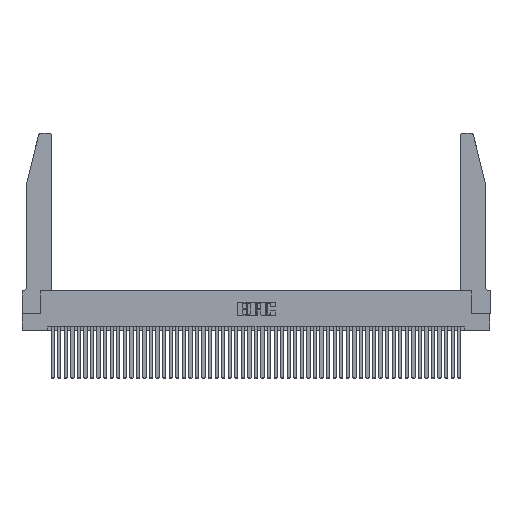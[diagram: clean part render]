
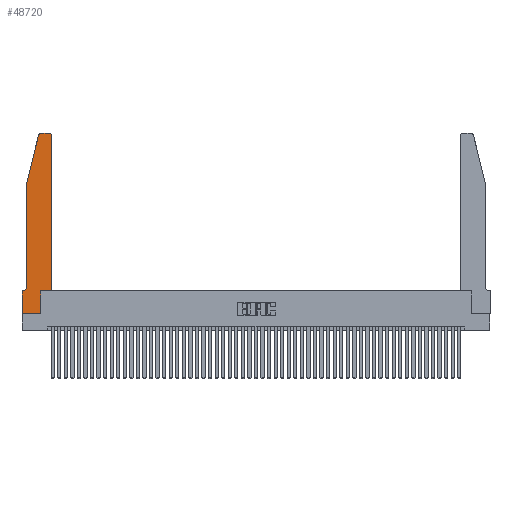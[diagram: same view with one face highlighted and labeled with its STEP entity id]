
A CAD part, top view. The second image highlights one B-rep face of the part: STEP entity #48720.
In plain terms, the highlighted planar face has unit normal (0, 0, 1).
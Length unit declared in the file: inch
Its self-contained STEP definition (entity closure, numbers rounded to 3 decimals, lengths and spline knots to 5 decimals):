
#128 = DIRECTION ( 'NONE',  ( 1., 0., 0. ) ) ;
#331 = CARTESIAN_POINT ( 'NONE',  ( 0.4505, 0.35, 0.37 ) ) ;
#742 = DIRECTION ( 'NONE',  ( -1., 0., 0. ) ) ;
#1206 = DIRECTION ( 'NONE',  ( 0., 1., 0. ) ) ;
#2209 = EDGE_CURVE ( 'NONE', #40006, #32432, #47138, .T. ) ;
#3001 = CARTESIAN_POINT ( 'NONE',  ( 0.0755, 2., 0.37 ) ) ;
#3090 = DIRECTION ( 'NONE',  ( 0., 0., 1. ) ) ;
#4704 = ORIENTED_EDGE ( 'NONE', *, *, #40652, .T. ) ;
#4999 = LINE ( 'NONE', #37681, #24915 ) ;
#5500 = DIRECTION ( 'NONE',  ( 1., 0., 0. ) ) ;
#5932 = AXIS2_PLACEMENT_3D ( 'NONE', #47526, #24015, #128 ) ;
#6295 = CARTESIAN_POINT ( 'NONE',  ( 0.284, 2.75, 0.37 ) ) ;
#7671 = CARTESIAN_POINT ( 'NONE',  ( 0.4505, 2.72, 0.37 ) ) ;
#7992 = VECTOR ( 'NONE', #13458, 39.37008 ) ;
#8046 = CARTESIAN_POINT ( 'NONE',  ( 0.0055, 0.42, 0.37 ) ) ;
#9437 = CARTESIAN_POINT ( 'NONE',  ( 0.0055, 0.35, 0.37 ) ) ;
#9988 = DIRECTION ( 'NONE',  ( 1., 0., 0. ) ) ;
#10695 = EDGE_CURVE ( 'NONE', #36535, #32628, #16369, .T. ) ;
#12051 = DIRECTION ( 'NONE',  ( -1., 0., 0. ) ) ;
#13458 = DIRECTION ( 'NONE',  ( -0.239, -0.971, 0. ) ) ;
#13918 = VERTEX_POINT ( 'NONE', #31488 ) ;
#13944 = EDGE_CURVE ( 'NONE', #13918, #24894, #30889, .T. ) ;
#14891 = CIRCLE ( 'NONE', #5932, 0.03 ) ;
#16247 = DIRECTION ( 'NONE',  ( 0., 1., 0. ) ) ;
#16369 = LINE ( 'NONE', #331, #21936 ) ;
#16769 = VECTOR ( 'NONE', #1206, 39.37008 ) ;
#17082 = CARTESIAN_POINT ( 'NONE',  ( 0.2865, 0., 0.37 ) ) ;
#17313 = ORIENTED_EDGE ( 'NONE', *, *, #24351, .T. ) ;
#17375 = DIRECTION ( 'NONE',  ( 0., 0., 1. ) ) ;
#17654 = ORIENTED_EDGE ( 'NONE', *, *, #47151, .T. ) ;
#17729 = ORIENTED_EDGE ( 'NONE', *, *, #24522, .T. ) ;
#20104 = AXIS2_PLACEMENT_3D ( 'NONE', #41002, #17375, #5500 ) ;
#21068 = LINE ( 'NONE', #43829, #48697 ) ;
#21235 = CARTESIAN_POINT ( 'NONE',  ( 0.4205, 2.75, 0.37 ) ) ;
#21766 = ORIENTED_EDGE ( 'NONE', *, *, #10695, .T. ) ;
#21936 = VECTOR ( 'NONE', #16247, 39.37008 ) ;
#22227 = ORIENTED_EDGE ( 'NONE', *, *, #43563, .T. ) ;
#22524 = EDGE_LOOP ( 'NONE', ( #30308, #22227, #4704, #17313, #17729, #45266, #46137, #46357, #17654, #35206, #21766, #42772 ) ) ;
#22870 = CARTESIAN_POINT ( 'NONE',  ( 0.25487, 2.72718, 0.37 ) ) ;
#24015 = DIRECTION ( 'NONE',  ( 0., 0., 1. ) ) ;
#24339 = VERTEX_POINT ( 'NONE', #22870 ) ;
#24351 = EDGE_CURVE ( 'NONE', #44704, #35537, #49083, .T. ) ;
#24522 = EDGE_CURVE ( 'NONE', #35537, #30404, #41735, .T. ) ;
#24894 = VERTEX_POINT ( 'NONE', #41754 ) ;
#24915 = VECTOR ( 'NONE', #9988, 39.37008 ) ;
#25075 = CARTESIAN_POINT ( 'NONE',  ( 0.2865, 0.35, 0.37 ) ) ;
#26059 = LINE ( 'NONE', #25075, #16769 ) ;
#26193 = EDGE_CURVE ( 'NONE', #24894, #32884, #4999, .T. ) ;
#26883 = DIRECTION ( 'NONE',  ( 0., -1., 0. ) ) ;
#26972 = CARTESIAN_POINT ( 'NONE',  ( 0.284, 2.72, 0.37 ) ) ;
#26978 = EDGE_CURVE ( 'NONE', #32628, #40006, #14891, .T. ) ;
#27227 = LINE ( 'NONE', #28622, #45606 ) ;
#28622 = CARTESIAN_POINT ( 'NONE',  ( 0.0755, 0.35, 0.37 ) ) ;
#28659 = DIRECTION ( 'NONE',  ( -1., 0., 0. ) ) ;
#28870 = AXIS2_PLACEMENT_3D ( 'NONE', #26972, #3090, #30916 ) ;
#30302 = CARTESIAN_POINT ( 'NONE',  ( 0.0755, 2., 0.37 ) ) ;
#30308 = ORIENTED_EDGE ( 'NONE', *, *, #2209, .T. ) ;
#30404 = VERTEX_POINT ( 'NONE', #9437 ) ;
#30889 = LINE ( 'NONE', #39538, #50454 ) ;
#30916 = DIRECTION ( 'NONE',  ( 1., 0., 0. ) ) ;
#31488 = CARTESIAN_POINT ( 'NONE',  ( 0., 0.35, 0.37 ) ) ;
#32432 = VERTEX_POINT ( 'NONE', #6295 ) ;
#32628 = VERTEX_POINT ( 'NONE', #7671 ) ;
#32884 = VERTEX_POINT ( 'NONE', #17082 ) ;
#33240 = CARTESIAN_POINT ( 'NONE',  ( 0.0755, 2., 0.37 ) ) ;
#35206 = ORIENTED_EDGE ( 'NONE', *, *, #41073, .T. ) ;
#35537 = VERTEX_POINT ( 'NONE', #47936 ) ;
#35781 = DIRECTION ( 'NONE',  ( 0., 0., -1. ) ) ;
#36535 = VERTEX_POINT ( 'NONE', #46717 ) ;
#36744 = VECTOR ( 'NONE', #28659, 39.37008 ) ;
#37458 = VECTOR ( 'NONE', #26883, 39.37008 ) ;
#37681 = CARTESIAN_POINT ( 'NONE',  ( 0., 0., 0.37 ) ) ;
#39403 = CIRCLE ( 'NONE', #28870, 0.03 ) ;
#39538 = CARTESIAN_POINT ( 'NONE',  ( 0., 0., 0.37 ) ) ;
#40006 = VERTEX_POINT ( 'NONE', #21235 ) ;
#40393 = AXIS2_PLACEMENT_3D ( 'NONE', #8046, #35781, #12051 ) ;
#40652 = EDGE_CURVE ( 'NONE', #24339, #44704, #48748, .T. ) ;
#41002 = CARTESIAN_POINT ( 'NONE',  ( 0., 0.35, 0.37 ) ) ;
#41073 = EDGE_CURVE ( 'NONE', #44469, #36535, #21068, .T. ) ;
#41735 = CIRCLE ( 'NONE', #40393, 0.07 ) ;
#41754 = CARTESIAN_POINT ( 'NONE',  ( 0., 0., 0.37 ) ) ;
#42506 = EDGE_CURVE ( 'NONE', #30404, #13918, #27227, .T. ) ;
#42772 = ORIENTED_EDGE ( 'NONE', *, *, #26978, .T. ) ;
#43485 = DIRECTION ( 'NONE',  ( 0., -1., 0. ) ) ;
#43563 = EDGE_CURVE ( 'NONE', #32432, #24339, #39403, .T. ) ;
#43829 = CARTESIAN_POINT ( 'NONE',  ( 0.4505, 0.35, 0.37 ) ) ;
#44256 = CARTESIAN_POINT ( 'NONE',  ( 0.2605, 2.75, 0.37 ) ) ;
#44469 = VERTEX_POINT ( 'NONE', #48629 ) ;
#44704 = VERTEX_POINT ( 'NONE', #30302 ) ;
#45266 = ORIENTED_EDGE ( 'NONE', *, *, #42506, .T. ) ;
#45606 = VECTOR ( 'NONE', #742, 39.37008 ) ;
#46137 = ORIENTED_EDGE ( 'NONE', *, *, #13944, .T. ) ;
#46357 = ORIENTED_EDGE ( 'NONE', *, *, #26193, .T. ) ;
#46717 = CARTESIAN_POINT ( 'NONE',  ( 0.4505, 0.35, 0.37 ) ) ;
#47138 = LINE ( 'NONE', #44256, #36744 ) ;
#47151 = EDGE_CURVE ( 'NONE', #32884, #44469, #26059, .T. ) ;
#47526 = CARTESIAN_POINT ( 'NONE',  ( 0.4205, 2.72, 0.37 ) ) ;
#47750 = DIRECTION ( 'NONE',  ( 1., 0., 0. ) ) ;
#47936 = CARTESIAN_POINT ( 'NONE',  ( 0.0755, 0.42, 0.37 ) ) ;
#48187 = FACE_OUTER_BOUND ( 'NONE', #22524, .T. ) ;
#48629 = CARTESIAN_POINT ( 'NONE',  ( 0.2865, 0.35, 0.37 ) ) ;
#48697 = VECTOR ( 'NONE', #47750, 39.37008 ) ;
#48720 = ADVANCED_FACE ( 'NONE', ( #48187 ), #48846, .T. ) ;
#48748 = LINE ( 'NONE', #33240, #7992 ) ;
#48846 = PLANE ( 'NONE',  #20104 ) ;
#49083 = LINE ( 'NONE', #3001, #37458 ) ;
#50454 = VECTOR ( 'NONE', #43485, 39.37008 ) ;
